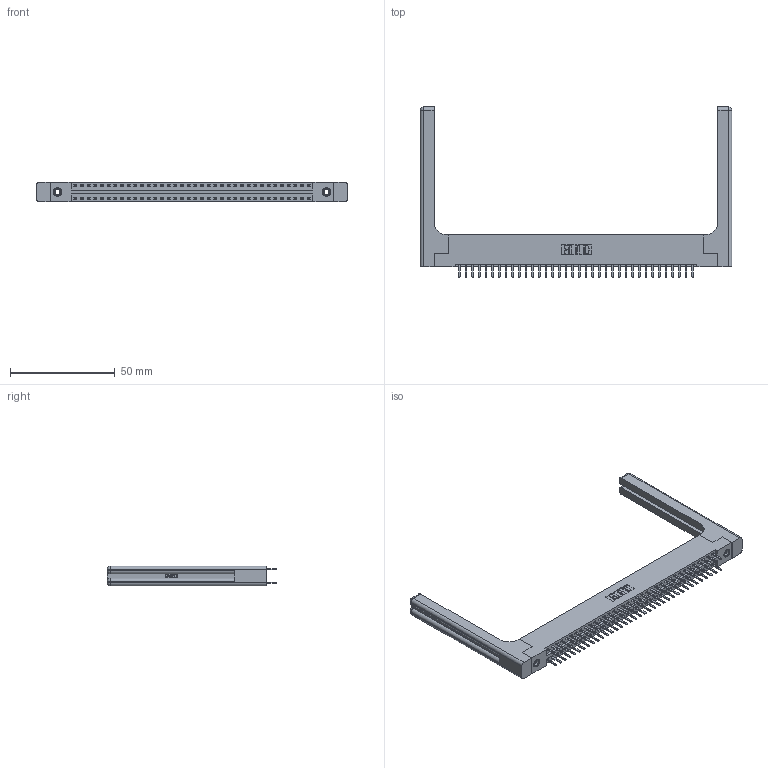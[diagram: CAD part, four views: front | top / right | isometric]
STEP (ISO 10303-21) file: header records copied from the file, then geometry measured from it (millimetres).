
FILE_DESCRIPTION (( 'STEP AP203' ), '1' );
FILE_NAME ('396-072-520-258.STEP', '2019-10-30T19:51:01', ( '' ), ( '' ), 'SwSTEP 2.0', 'SolidWorks 2016', '' );
FILE_SCHEMA (( 'CONFIG_CONTROL_DESIGN' ));
Length unit declared in the file: inch
Products named in the file (5): 396-072-520-258; 345-250-001_345-250-001-102; 346 Part_Flush Mounting Lugs - 0.156 Dia-TH; 346-220-058_345-220-058; 345-292-001_345-293-120
Assembly tree (77 placements, depth 2):
  396-072-520-258
    346 Part_Flush Mounting Lugs - 0.156 Dia-TH
    345-292-001_345-293-120  x72
    345-250-001_345-250-001-102  x2
    346-220-058_345-220-058  x2
Bounding box: 148.36 x 80.98 x 9.4 mm (x, y, z)
Volume: 21883.1 mm3; surface area: 24582.7 mm2
Topology: 77 solids, 77 shells, 4410 faces, 12731 edges, 8274 vertices
Faces by surface type: plane 2888, cylinder 1462, bspline 36, cone 12, sphere 8, torus 4
Entity records: 29598 total; most frequent: CARTESIAN_POINT 5905, ORIENTED_EDGE 4624, DIRECTION 4176, EDGE_CURVE 2312, LINE 1940, VECTOR 1940, VERTEX_POINT 1530, AXIS2_PLACEMENT_3D 1118
